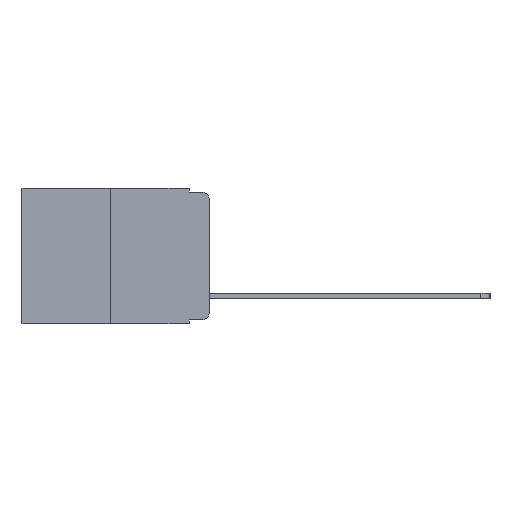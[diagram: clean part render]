
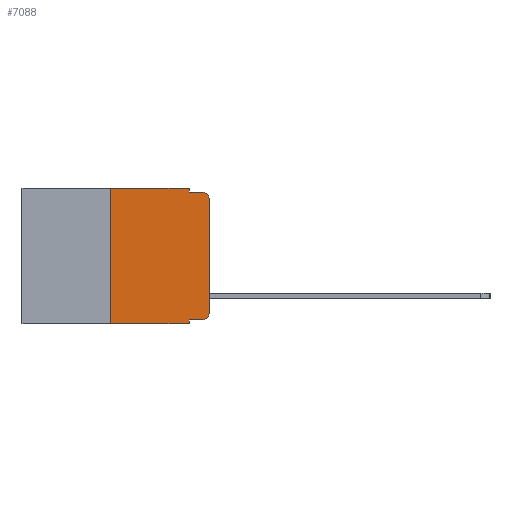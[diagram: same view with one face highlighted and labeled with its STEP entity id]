
A CAD part, left-side view. The second image highlights one B-rep face of the part: STEP entity #7088.
In plain terms, the highlighted planar face has unit normal (-1, 0, 0).
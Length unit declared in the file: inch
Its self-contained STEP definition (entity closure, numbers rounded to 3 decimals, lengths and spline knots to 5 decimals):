
#302 = VECTOR ( 'NONE', #5671, 39.37008 ) ;
#411 = VERTEX_POINT ( 'NONE', #11002 ) ;
#843 = VERTEX_POINT ( 'NONE', #1659 ) ;
#1125 = VECTOR ( 'NONE', #8335, 39.37008 ) ;
#1659 = CARTESIAN_POINT ( 'NONE',  ( 0., 0.051, -0.343 ) ) ;
#1680 = VERTEX_POINT ( 'NONE', #6706 ) ;
#1971 = EDGE_LOOP ( 'NONE', ( #2321, #2648, #2684, #2709, #2760, #3082, #3105, #3120, #3244, #3330 ) ) ;
#2075 = VERTEX_POINT ( 'NONE', #9562 ) ;
#2195 = LINE ( 'NONE', #4782, #12748 ) ;
#2209 = DIRECTION ( 'NONE',  ( 1., 0., 0. ) ) ;
#2321 = ORIENTED_EDGE ( 'NONE', *, *, #11591, .T. ) ;
#2498 = CARTESIAN_POINT ( 'NONE',  ( 0., 0., -0.313 ) ) ;
#2625 = FACE_OUTER_BOUND ( 'NONE', #1971, .T. ) ;
#2648 = ORIENTED_EDGE ( 'NONE', *, *, #10933, .T. ) ;
#2684 = ORIENTED_EDGE ( 'NONE', *, *, #10281, .F. ) ;
#2709 = ORIENTED_EDGE ( 'NONE', *, *, #9617, .F. ) ;
#2760 = ORIENTED_EDGE ( 'NONE', *, *, #9677, .F. ) ;
#2793 = CARTESIAN_POINT ( 'NONE',  ( 0., 0.051, 0. ) ) ;
#2844 = LINE ( 'NONE', #7316, #13331 ) ;
#2845 = AXIS2_PLACEMENT_3D ( 'NONE', #12329, #12389, #12568 ) ;
#2925 = VECTOR ( 'NONE', #4073, 39.37008 ) ;
#3082 = ORIENTED_EDGE ( 'NONE', *, *, #8232, .F. ) ;
#3105 = ORIENTED_EDGE ( 'NONE', *, *, #13351, .T. ) ;
#3120 = ORIENTED_EDGE ( 'NONE', *, *, #7482, .F. ) ;
#3244 = ORIENTED_EDGE ( 'NONE', *, *, #5932, .T. ) ;
#3330 = ORIENTED_EDGE ( 'NONE', *, *, #4519, .T. ) ;
#3350 = LINE ( 'NONE', #10034, #302 ) ;
#3395 = CARTESIAN_POINT ( 'NONE',  ( 0., 0.02, -0.333 ) ) ;
#3861 = DIRECTION ( 'NONE',  ( -1., 0., 0. ) ) ;
#4073 = DIRECTION ( 'NONE',  ( 0., 0., 1. ) ) ;
#4078 = LINE ( 'NONE', #12299, #1125 ) ;
#4519 = EDGE_CURVE ( 'NONE', #8002, #13398, #5701, .T. ) ;
#4782 = CARTESIAN_POINT ( 'NONE',  ( 0., 0.051, -0.01 ) ) ;
#4880 = DIRECTION ( 'NONE',  ( 0., 0., -1. ) ) ;
#5346 = CARTESIAN_POINT ( 'NONE',  ( 0., 0.473, 0. ) ) ;
#5671 = DIRECTION ( 'NONE',  ( 0., -1., 0. ) ) ;
#5701 = CIRCLE ( 'NONE', #2845, 0.02 ) ;
#5932 = EDGE_CURVE ( 'NONE', #13771, #8002, #2844, .T. ) ;
#6129 = CARTESIAN_POINT ( 'NONE',  ( 0., 0.051, -0.333 ) ) ;
#6706 = CARTESIAN_POINT ( 'NONE',  ( 0., 0.25, -0.343 ) ) ;
#6965 = AXIS2_PLACEMENT_3D ( 'NONE', #10265, #3861, #11251 ) ;
#7088 = ADVANCED_FACE ( 'NONE', ( #2625 ), #10703, .F. ) ;
#7316 = CARTESIAN_POINT ( 'NONE',  ( 0., 0.051, -0.333 ) ) ;
#7482 = EDGE_CURVE ( 'NONE', #13771, #843, #13444, .T. ) ;
#7699 = VECTOR ( 'NONE', #12255, 39.37008 ) ;
#8002 = VERTEX_POINT ( 'NONE', #3395 ) ;
#8032 = LINE ( 'NONE', #2793, #7699 ) ;
#8232 = EDGE_CURVE ( 'NONE', #1680, #9959, #11073, .T. ) ;
#8335 = DIRECTION ( 'NONE',  ( 0., -1., 0. ) ) ;
#8441 = DIRECTION ( 'NONE',  ( 0., -1., 0. ) ) ;
#8518 = CIRCLE ( 'NONE', #6965, 0.02 ) ;
#8698 = CARTESIAN_POINT ( 'NONE',  ( 0., 0.25, 0. ) ) ;
#9562 = CARTESIAN_POINT ( 'NONE',  ( 0., 0.02, -0.01 ) ) ;
#9617 = EDGE_CURVE ( 'NONE', #411, #12541, #8032, .T. ) ;
#9618 = VECTOR ( 'NONE', #10079, 39.37008 ) ;
#9677 = EDGE_CURVE ( 'NONE', #9959, #411, #4078, .T. ) ;
#9773 = DIRECTION ( 'NONE',  ( 0., 0., -1. ) ) ;
#9959 = VERTEX_POINT ( 'NONE', #8698 ) ;
#10034 = CARTESIAN_POINT ( 'NONE',  ( 0., 0.473, -0.343 ) ) ;
#10079 = DIRECTION ( 'NONE',  ( 0., 0., 1. ) ) ;
#10103 = CARTESIAN_POINT ( 'NONE',  ( 0., 0.051, -0.01 ) ) ;
#10265 = CARTESIAN_POINT ( 'NONE',  ( 0., 0.02, -0.03 ) ) ;
#10281 = EDGE_CURVE ( 'NONE', #12541, #2075, #2195, .T. ) ;
#10467 = CARTESIAN_POINT ( 'NONE',  ( 0., 0.25, 0. ) ) ;
#10703 = PLANE ( 'NONE',  #11918 ) ;
#10933 = EDGE_CURVE ( 'NONE', #12094, #2075, #8518, .T. ) ;
#11002 = CARTESIAN_POINT ( 'NONE',  ( 0., 0.051, 0. ) ) ;
#11073 = LINE ( 'NONE', #10467, #2925 ) ;
#11251 = DIRECTION ( 'NONE',  ( 0., 0., -1. ) ) ;
#11591 = EDGE_CURVE ( 'NONE', #13398, #12094, #12546, .T. ) ;
#11656 = CARTESIAN_POINT ( 'NONE',  ( 0., 0., -0.03 ) ) ;
#11918 = AXIS2_PLACEMENT_3D ( 'NONE', #5346, #2209, #9773 ) ;
#12004 = CARTESIAN_POINT ( 'NONE',  ( 0., 0., 0. ) ) ;
#12094 = VERTEX_POINT ( 'NONE', #11656 ) ;
#12255 = DIRECTION ( 'NONE',  ( 0., 0., -1. ) ) ;
#12264 = CARTESIAN_POINT ( 'NONE',  ( 0., 0.051, 0. ) ) ;
#12299 = CARTESIAN_POINT ( 'NONE',  ( 0., 0.473, 0. ) ) ;
#12329 = CARTESIAN_POINT ( 'NONE',  ( 0., 0.02, -0.313 ) ) ;
#12389 = DIRECTION ( 'NONE',  ( -1., 0., 0. ) ) ;
#12541 = VERTEX_POINT ( 'NONE', #10103 ) ;
#12546 = LINE ( 'NONE', #12004, #9618 ) ;
#12568 = DIRECTION ( 'NONE',  ( 0., 0., -1. ) ) ;
#12748 = VECTOR ( 'NONE', #13179, 39.37008 ) ;
#13139 = VECTOR ( 'NONE', #4880, 39.37008 ) ;
#13179 = DIRECTION ( 'NONE',  ( 0., -1., 0. ) ) ;
#13331 = VECTOR ( 'NONE', #8441, 39.37008 ) ;
#13351 = EDGE_CURVE ( 'NONE', #1680, #843, #3350, .T. ) ;
#13398 = VERTEX_POINT ( 'NONE', #2498 ) ;
#13444 = LINE ( 'NONE', #12264, #13139 ) ;
#13771 = VERTEX_POINT ( 'NONE', #6129 ) ;
